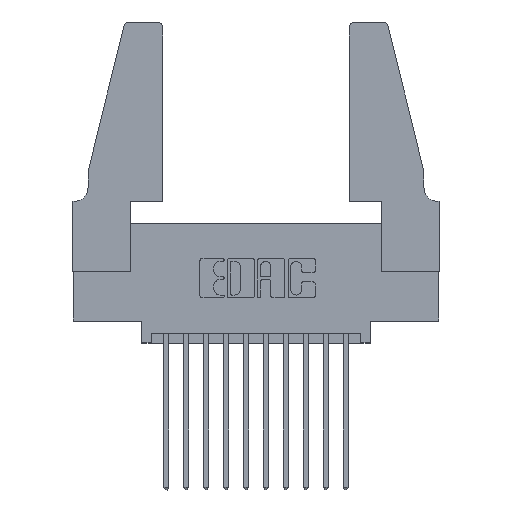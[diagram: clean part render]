
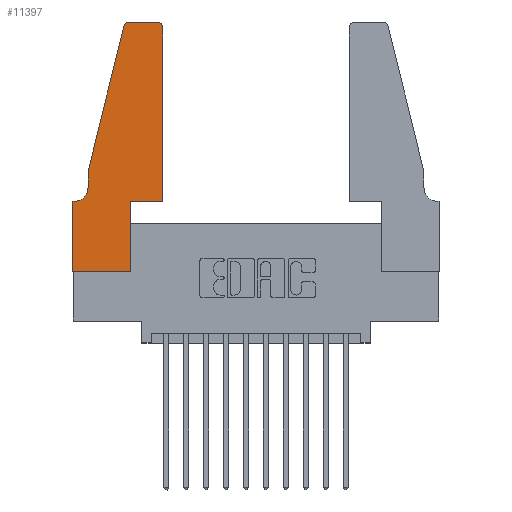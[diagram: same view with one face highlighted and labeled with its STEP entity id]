
A CAD part, top view. The second image highlights one B-rep face of the part: STEP entity #11397.
In plain terms, the highlighted planar face has unit normal (0, 0, 1).
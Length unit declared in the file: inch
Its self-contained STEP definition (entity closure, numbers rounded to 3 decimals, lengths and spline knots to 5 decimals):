
#21 = ORIENTED_EDGE ( 'NONE', *, *, #11395, .T. ) ;
#98 = VECTOR ( 'NONE', #10864, 39.37008 ) ;
#455 = EDGE_CURVE ( 'NONE', #12055, #3900, #9511, .T. ) ;
#477 = LINE ( 'NONE', #8774, #7657 ) ;
#549 = CARTESIAN_POINT ( 'NONE',  ( 0.4505, 0.35, 0.37 ) ) ;
#662 = VERTEX_POINT ( 'NONE', #2922 ) ;
#1024 = CARTESIAN_POINT ( 'NONE',  ( 0.284, 1.22, 0.37 ) ) ;
#1067 = DIRECTION ( 'NONE',  ( 0., 1., 0. ) ) ;
#1181 = ORIENTED_EDGE ( 'NONE', *, *, #5203, .T. ) ;
#1505 = VERTEX_POINT ( 'NONE', #7842 ) ;
#1676 = AXIS2_PLACEMENT_3D ( 'NONE', #4902, #13871, #9263 ) ;
#1781 = EDGE_CURVE ( 'NONE', #10582, #662, #11709, .T. ) ;
#2162 = VECTOR ( 'NONE', #5039, 39.37008 ) ;
#2254 = CARTESIAN_POINT ( 'NONE',  ( 0.0755, 0.5, 0.37 ) ) ;
#2505 = DIRECTION ( 'NONE',  ( -0.239, -0.971, 0. ) ) ;
#2652 = VECTOR ( 'NONE', #12506, 39.37008 ) ;
#2693 = LINE ( 'NONE', #9649, #14273 ) ;
#2922 = CARTESIAN_POINT ( 'NONE',  ( 0.0055, 0.35, 0.37 ) ) ;
#3050 = AXIS2_PLACEMENT_3D ( 'NONE', #10437, #13870, #5961 ) ;
#3150 = CARTESIAN_POINT ( 'NONE',  ( 0.0755, 0.35, 0.37 ) ) ;
#3418 = ORIENTED_EDGE ( 'NONE', *, *, #4812, .T. ) ;
#3695 = VERTEX_POINT ( 'NONE', #549 ) ;
#3743 = LINE ( 'NONE', #13274, #12136 ) ;
#3900 = VERTEX_POINT ( 'NONE', #2254 ) ;
#3970 = VERTEX_POINT ( 'NONE', #7895 ) ;
#4223 = DIRECTION ( 'NONE',  ( 0., 0., 1. ) ) ;
#4812 = EDGE_CURVE ( 'NONE', #11696, #7066, #3743, .T. ) ;
#4902 = CARTESIAN_POINT ( 'NONE',  ( 0.4205, 1.22, 0.37 ) ) ;
#5039 = DIRECTION ( 'NONE',  ( 0., -1., 0. ) ) ;
#5077 = EDGE_CURVE ( 'NONE', #3695, #10244, #2693, .T. ) ;
#5105 = LINE ( 'NONE', #3150, #11738 ) ;
#5203 = EDGE_CURVE ( 'NONE', #1505, #8791, #9515, .T. ) ;
#5400 = DIRECTION ( 'NONE',  ( -1., 0., 0. ) ) ;
#5738 = EDGE_CURVE ( 'NONE', #3970, #11696, #7230, .T. ) ;
#5806 = EDGE_CURVE ( 'NONE', #7066, #3695, #13867, .T. ) ;
#5858 = CARTESIAN_POINT ( 'NONE',  ( 0.0755, 0.42, 0.37 ) ) ;
#5899 = ORIENTED_EDGE ( 'NONE', *, *, #9253, .T. ) ;
#5961 = DIRECTION ( 'NONE',  ( 1., 0., 0. ) ) ;
#6035 = CARTESIAN_POINT ( 'NONE',  ( 0.2865, 0.35, 0.37 ) ) ;
#6039 = VECTOR ( 'NONE', #2505, 39.37008 ) ;
#6072 = VERTEX_POINT ( 'NONE', #12939 ) ;
#6158 = PLANE ( 'NONE',  #3050 ) ;
#6316 = CARTESIAN_POINT ( 'NONE',  ( 0.4505, 1.22, 0.37 ) ) ;
#6575 = EDGE_LOOP ( 'NONE', ( #1181, #7208, #8008, #5899, #10558, #7803, #21, #12206, #3418, #8433, #7828, #10045 ) ) ;
#6794 = CARTESIAN_POINT ( 'NONE',  ( 0.0055, 0.42, 0.37 ) ) ;
#6842 = CARTESIAN_POINT ( 'NONE',  ( 0., 0., 0.37 ) ) ;
#7055 = CARTESIAN_POINT ( 'NONE',  ( 0.284, 1.25, 0.37 ) ) ;
#7066 = VERTEX_POINT ( 'NONE', #6035 ) ;
#7208 = ORIENTED_EDGE ( 'NONE', *, *, #7830, .T. ) ;
#7230 = LINE ( 'NONE', #6842, #10361 ) ;
#7421 = EDGE_CURVE ( 'NONE', #662, #6072, #5105, .T. ) ;
#7607 = FACE_OUTER_BOUND ( 'NONE', #6575, .T. ) ;
#7657 = VECTOR ( 'NONE', #12030, 39.37008 ) ;
#7666 = EDGE_CURVE ( 'NONE', #10244, #1505, #11922, .T. ) ;
#7803 = ORIENTED_EDGE ( 'NONE', *, *, #7421, .T. ) ;
#7828 = ORIENTED_EDGE ( 'NONE', *, *, #5077, .T. ) ;
#7830 = EDGE_CURVE ( 'NONE', #8791, #12055, #8731, .T. ) ;
#7842 = CARTESIAN_POINT ( 'NONE',  ( 0.4205, 1.25, 0.37 ) ) ;
#7895 = CARTESIAN_POINT ( 'NONE',  ( 0., 0., 0.37 ) ) ;
#8008 = ORIENTED_EDGE ( 'NONE', *, *, #455, .T. ) ;
#8063 = AXIS2_PLACEMENT_3D ( 'NONE', #6794, #8842, #8975 ) ;
#8433 = ORIENTED_EDGE ( 'NONE', *, *, #5806, .T. ) ;
#8469 = LINE ( 'NONE', #9460, #2162 ) ;
#8731 = CIRCLE ( 'NONE', #13399, 0.03 ) ;
#8774 = CARTESIAN_POINT ( 'NONE',  ( 0.0755, 0.5, 0.37 ) ) ;
#8791 = VERTEX_POINT ( 'NONE', #7055 ) ;
#8842 = DIRECTION ( 'NONE',  ( 0., 0., -1. ) ) ;
#8975 = DIRECTION ( 'NONE',  ( -1., 0., 0. ) ) ;
#9253 = EDGE_CURVE ( 'NONE', #3900, #10582, #477, .T. ) ;
#9263 = DIRECTION ( 'NONE',  ( 1., 0., 0. ) ) ;
#9460 = CARTESIAN_POINT ( 'NONE',  ( 0., 0., 0.37 ) ) ;
#9511 = LINE ( 'NONE', #11523, #6039 ) ;
#9515 = LINE ( 'NONE', #14265, #98 ) ;
#9649 = CARTESIAN_POINT ( 'NONE',  ( 0.4505, 0.35, 0.37 ) ) ;
#10045 = ORIENTED_EDGE ( 'NONE', *, *, #7666, .T. ) ;
#10244 = VERTEX_POINT ( 'NONE', #6316 ) ;
#10340 = CARTESIAN_POINT ( 'NONE',  ( 0.4505, 0.35, 0.37 ) ) ;
#10361 = VECTOR ( 'NONE', #11135, 39.37008 ) ;
#10437 = CARTESIAN_POINT ( 'NONE',  ( 0., 0.35, 0.37 ) ) ;
#10558 = ORIENTED_EDGE ( 'NONE', *, *, #1781, .T. ) ;
#10582 = VERTEX_POINT ( 'NONE', #5858 ) ;
#10864 = DIRECTION ( 'NONE',  ( -1., 0., 0. ) ) ;
#11135 = DIRECTION ( 'NONE',  ( 1., 0., 0. ) ) ;
#11395 = EDGE_CURVE ( 'NONE', #6072, #3970, #8469, .T. ) ;
#11397 = ADVANCED_FACE ( 'NONE', ( #7607 ), #6158, .T. ) ;
#11523 = CARTESIAN_POINT ( 'NONE',  ( 0.0755, 0.5, 0.37 ) ) ;
#11567 = CARTESIAN_POINT ( 'NONE',  ( 0.25487, 1.22718, 0.37 ) ) ;
#11696 = VERTEX_POINT ( 'NONE', #12696 ) ;
#11709 = CIRCLE ( 'NONE', #8063, 0.07 ) ;
#11738 = VECTOR ( 'NONE', #5400, 39.37008 ) ;
#11764 = DIRECTION ( 'NONE',  ( 0., 1., 0. ) ) ;
#11922 = CIRCLE ( 'NONE', #1676, 0.03 ) ;
#12030 = DIRECTION ( 'NONE',  ( 0., -1., 0. ) ) ;
#12055 = VERTEX_POINT ( 'NONE', #11567 ) ;
#12136 = VECTOR ( 'NONE', #1067, 39.37008 ) ;
#12206 = ORIENTED_EDGE ( 'NONE', *, *, #5738, .T. ) ;
#12506 = DIRECTION ( 'NONE',  ( 1., 0., 0. ) ) ;
#12696 = CARTESIAN_POINT ( 'NONE',  ( 0.2865, 0., 0.37 ) ) ;
#12939 = CARTESIAN_POINT ( 'NONE',  ( 0., 0.35, 0.37 ) ) ;
#13274 = CARTESIAN_POINT ( 'NONE',  ( 0.2865, 0.35, 0.37 ) ) ;
#13399 = AXIS2_PLACEMENT_3D ( 'NONE', #1024, #4223, #14227 ) ;
#13867 = LINE ( 'NONE', #10340, #2652 ) ;
#13870 = DIRECTION ( 'NONE',  ( 0., 0., 1. ) ) ;
#13871 = DIRECTION ( 'NONE',  ( 0., 0., 1. ) ) ;
#14227 = DIRECTION ( 'NONE',  ( 1., 0., 0. ) ) ;
#14265 = CARTESIAN_POINT ( 'NONE',  ( 0.2605, 1.25, 0.37 ) ) ;
#14273 = VECTOR ( 'NONE', #11764, 39.37008 ) ;
